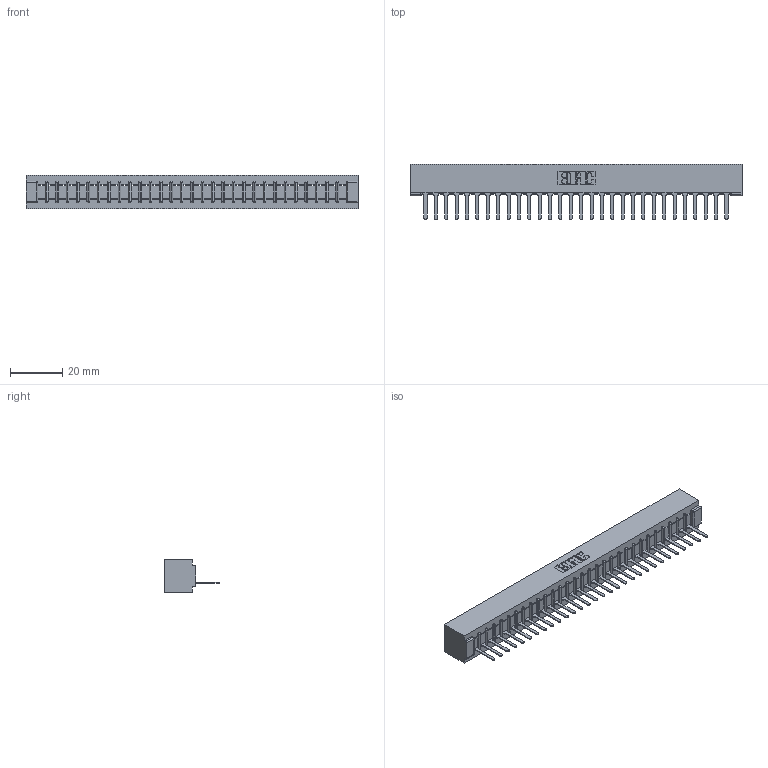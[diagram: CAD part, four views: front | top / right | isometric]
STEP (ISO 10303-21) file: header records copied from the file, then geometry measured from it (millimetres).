
FILE_DESCRIPTION (( 'STEP AP203' ), '1' );
FILE_NAME ('307-030-427-101.STEP', '2020-09-28T10:34:05', ( '' ), ( '' ), 'SwSTEP 2.0', 'SolidWorks 2020', '' );
FILE_SCHEMA (( 'CONFIG_CONTROL_DESIGN' ));
Length unit declared in the file: inch
Products named in the file (3): 307 Part_No Mounting Lugs; 307-030-427-101; 307-290-001_527
Assembly tree (31 placements, depth 2):
  307-030-427-101
    307 Part_No Mounting Lugs
    307-290-001_527  x30
Bounding box: 126.75 x 21.11 x 12.7 mm (x, y, z)
Volume: 13618 mm3; surface area: 14521.3 mm2
Topology: 31 solids, 31 shells, 1821 faces, 5159 edges, 3314 vertices
Faces by surface type: plane 1176, cylinder 583, sphere 62
Entity records: 26888 total; most frequent: CARTESIAN_POINT 4524, ORIENTED_EDGE 4510, DIRECTION 4405, EDGE_CURVE 2255, LINE 1727, VECTOR 1727, VERTEX_POINT 1458, AXIS2_PLACEMENT_3D 1339
